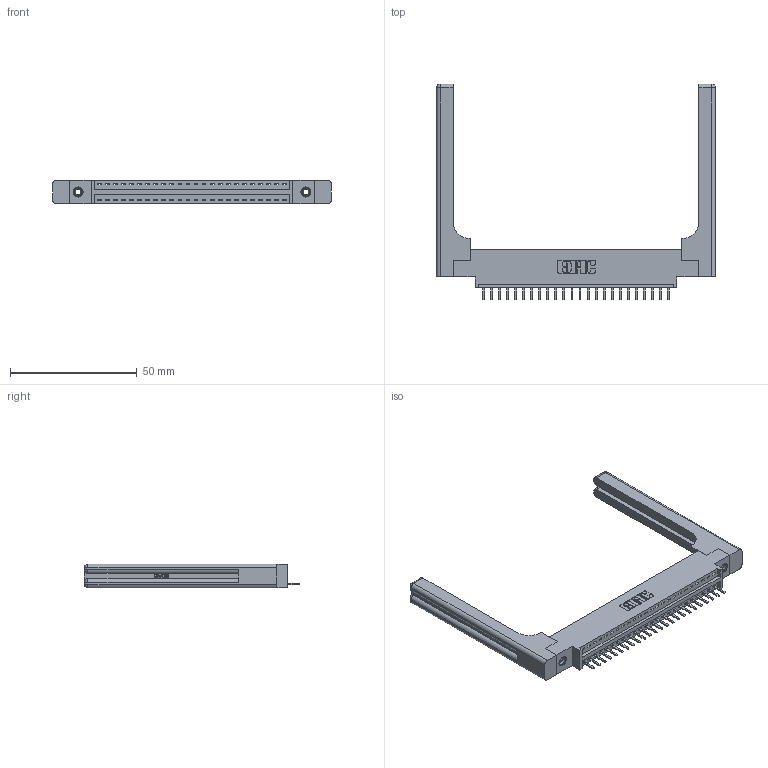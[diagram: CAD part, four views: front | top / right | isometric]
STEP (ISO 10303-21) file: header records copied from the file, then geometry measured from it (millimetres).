
FILE_DESCRIPTION (( 'STEP AP203' ), '1' );
FILE_NAME ('396-024-520-658.STEP', '2019-10-27T05:37:59', ( '' ), ( '' ), 'SwSTEP 2.0', 'SolidWorks 2016', '' );
FILE_SCHEMA (( 'CONFIG_CONTROL_DESIGN' ));
Length unit declared in the file: inch
Products named in the file (5): 396-024-520-658; 346-220-058_345-220-058; 345-250-001_345-250-001-102; 346 Part_0.170 Offset - 0.156 Dia-TH; 345-292-001_345-293-120
Assembly tree (29 placements, depth 2):
  396-024-520-658
    346 Part_0.170 Offset - 0.156 Dia-TH
    345-292-001_345-293-120  x24
    345-250-001_345-250-001-102  x2
    346-220-058_345-220-058  x2
Bounding box: 110.26 x 85.29 x 9.4 mm (x, y, z)
Volume: 17725.2 mm3; surface area: 17662.4 mm2
Topology: 29 solids, 29 shells, 1870 faces, 5423 edges, 3530 vertices
Faces by surface type: plane 1236, cylinder 574, bspline 36, cone 12, sphere 8, torus 4
Entity records: 22746 total; most frequent: CARTESIAN_POINT 4897, ORIENTED_EDGE 3640, DIRECTION 3260, EDGE_CURVE 1820, VECTOR 1496, LINE 1496, VERTEX_POINT 1202, AXIS2_PLACEMENT_3D 882
